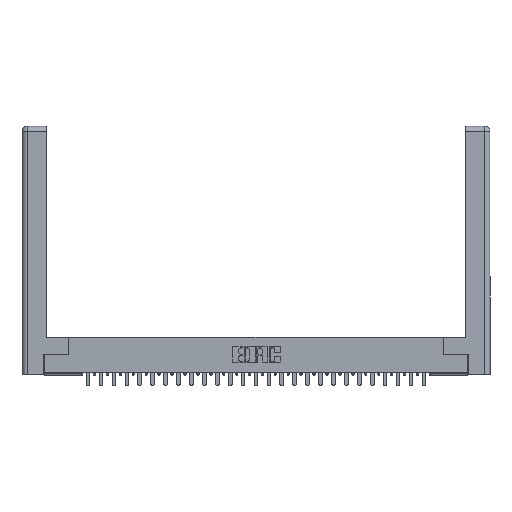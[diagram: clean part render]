
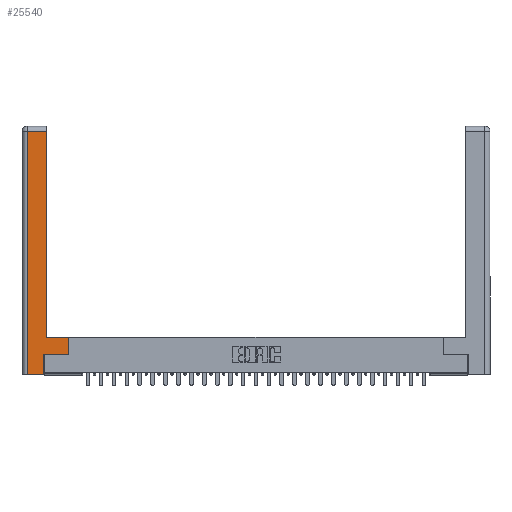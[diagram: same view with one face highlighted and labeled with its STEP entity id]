
A CAD part, top view. The second image highlights one B-rep face of the part: STEP entity #25540.
In plain terms, the highlighted planar face has unit normal (0, 0, 1).
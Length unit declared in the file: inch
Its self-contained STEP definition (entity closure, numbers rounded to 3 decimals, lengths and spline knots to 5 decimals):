
#487 = CARTESIAN_POINT ( 'NONE',  ( 0.565, 0.45, 0. ) ) ;
#734 = DIRECTION ( 'NONE',  ( -1., 0., 0. ) ) ;
#1129 = EDGE_CURVE ( 'NONE', #13912, #26344, #26014, .T. ) ;
#4277 = FACE_OUTER_BOUND ( 'NONE', #28629, .T. ) ;
#4902 = ORIENTED_EDGE ( 'NONE', *, *, #1129, .T. ) ;
#6026 = VERTEX_POINT ( 'NONE', #22496 ) ;
#6080 = LINE ( 'NONE', #16136, #12134 ) ;
#6691 = CARTESIAN_POINT ( 'NONE',  ( 0.265, 0.245, 0. ) ) ;
#6807 = CARTESIAN_POINT ( 'NONE',  ( 0.265, 0.245, 0. ) ) ;
#7443 = VECTOR ( 'NONE', #25118, 39.37008 ) ;
#8664 = LINE ( 'NONE', #31898, #13533 ) ;
#9012 = LINE ( 'NONE', #16829, #26528 ) ;
#9311 = DIRECTION ( 'NONE',  ( 0., 1., 0. ) ) ;
#9451 = LINE ( 'NONE', #26767, #18832 ) ;
#10478 = AXIS2_PLACEMENT_3D ( 'NONE', #29991, #11798, #11575 ) ;
#10575 = DIRECTION ( 'NONE',  ( 0., 1., 0. ) ) ;
#10588 = VERTEX_POINT ( 'NONE', #6691 ) ;
#11245 = DIRECTION ( 'NONE',  ( 0., -1., 0. ) ) ;
#11575 = DIRECTION ( 'NONE',  ( -1., 0., 0. ) ) ;
#11798 = DIRECTION ( 'NONE',  ( 0., 0., -1. ) ) ;
#12134 = VECTOR ( 'NONE', #11245, 39.37008 ) ;
#12828 = CARTESIAN_POINT ( 'NONE',  ( 0.565, 0.45, 0. ) ) ;
#13414 = VECTOR ( 'NONE', #20549, 39.37008 ) ;
#13533 = VECTOR ( 'NONE', #734, 39.37008 ) ;
#13912 = VERTEX_POINT ( 'NONE', #21538 ) ;
#16039 = DIRECTION ( 'NONE',  ( 1., 0., 0. ) ) ;
#16136 = CARTESIAN_POINT ( 'NONE',  ( 0.0615, 0., 0. ) ) ;
#16802 = VECTOR ( 'NONE', #10575, 39.37008 ) ;
#16829 = CARTESIAN_POINT ( 'NONE',  ( 0.0615, 2.94, 0. ) ) ;
#18485 = CARTESIAN_POINT ( 'NONE',  ( 0.565, 0.245, 0. ) ) ;
#18832 = VECTOR ( 'NONE', #16039, 39.37008 ) ;
#19325 = VERTEX_POINT ( 'NONE', #25917 ) ;
#19525 = CARTESIAN_POINT ( 'NONE',  ( 0.295, 2.94, 0. ) ) ;
#20549 = DIRECTION ( 'NONE',  ( 1., 0., 0. ) ) ;
#20887 = CARTESIAN_POINT ( 'NONE',  ( 0.265, 0., 0. ) ) ;
#21538 = CARTESIAN_POINT ( 'NONE',  ( 0.295, 0.45, 0. ) ) ;
#21659 = ORIENTED_EDGE ( 'NONE', *, *, #29800, .T. ) ;
#22496 = CARTESIAN_POINT ( 'NONE',  ( 0.0615, 2.94, 0. ) ) ;
#23429 = ORIENTED_EDGE ( 'NONE', *, *, #28994, .T. ) ;
#24577 = PLANE ( 'NONE',  #10478 ) ;
#24593 = DIRECTION ( 'NONE',  ( -1., 0., 0. ) ) ;
#24848 = VERTEX_POINT ( 'NONE', #31207 ) ;
#24924 = VERTEX_POINT ( 'NONE', #487 ) ;
#25118 = DIRECTION ( 'NONE',  ( 0., 1., 0. ) ) ;
#25540 = ADVANCED_FACE ( 'NONE', ( #4277 ), #24577, .F. ) ;
#25917 = CARTESIAN_POINT ( 'NONE',  ( 0.265, 0., 0. ) ) ;
#26014 = LINE ( 'NONE', #27845, #27182 ) ;
#26344 = VERTEX_POINT ( 'NONE', #19525 ) ;
#26371 = ORIENTED_EDGE ( 'NONE', *, *, #31987, .T. ) ;
#26464 = LINE ( 'NONE', #20887, #13414 ) ;
#26528 = VECTOR ( 'NONE', #24593, 39.37008 ) ;
#26767 = CARTESIAN_POINT ( 'NONE',  ( 0.565, 0.245, 0. ) ) ;
#27182 = VECTOR ( 'NONE', #9311, 39.37008 ) ;
#27829 = LINE ( 'NONE', #12828, #16802 ) ;
#27845 = CARTESIAN_POINT ( 'NONE',  ( 0.295, 3., 0. ) ) ;
#28187 = LINE ( 'NONE', #6807, #7443 ) ;
#28546 = ORIENTED_EDGE ( 'NONE', *, *, #29092, .T. ) ;
#28569 = ORIENTED_EDGE ( 'NONE', *, *, #29375, .T. ) ;
#28629 = EDGE_LOOP ( 'NONE', ( #4902, #21659, #26371, #31561, #28569, #32255, #23429, #28546 ) ) ;
#28994 = EDGE_CURVE ( 'NONE', #32814, #24924, #27829, .T. ) ;
#29092 = EDGE_CURVE ( 'NONE', #24924, #13912, #8664, .T. ) ;
#29375 = EDGE_CURVE ( 'NONE', #19325, #10588, #28187, .T. ) ;
#29668 = EDGE_CURVE ( 'NONE', #10588, #32814, #9451, .T. ) ;
#29800 = EDGE_CURVE ( 'NONE', #26344, #6026, #9012, .T. ) ;
#29991 = CARTESIAN_POINT ( 'NONE',  ( 0., 0., 0. ) ) ;
#31153 = EDGE_CURVE ( 'NONE', #24848, #19325, #26464, .T. ) ;
#31207 = CARTESIAN_POINT ( 'NONE',  ( 0.0615, 0., 0. ) ) ;
#31561 = ORIENTED_EDGE ( 'NONE', *, *, #31153, .T. ) ;
#31898 = CARTESIAN_POINT ( 'NONE',  ( 0.295, 0.45, 0. ) ) ;
#31987 = EDGE_CURVE ( 'NONE', #6026, #24848, #6080, .T. ) ;
#32255 = ORIENTED_EDGE ( 'NONE', *, *, #29668, .T. ) ;
#32814 = VERTEX_POINT ( 'NONE', #18485 ) ;
